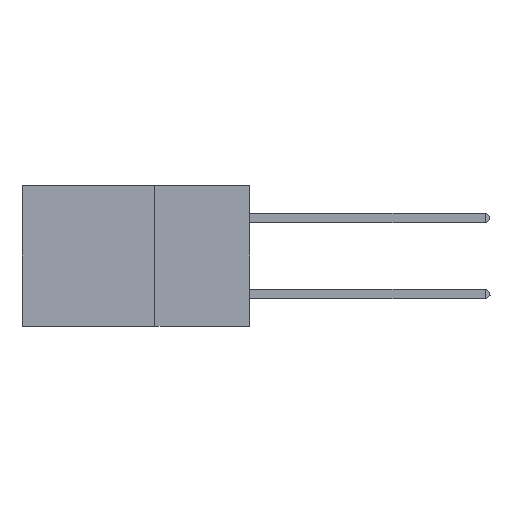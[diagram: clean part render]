
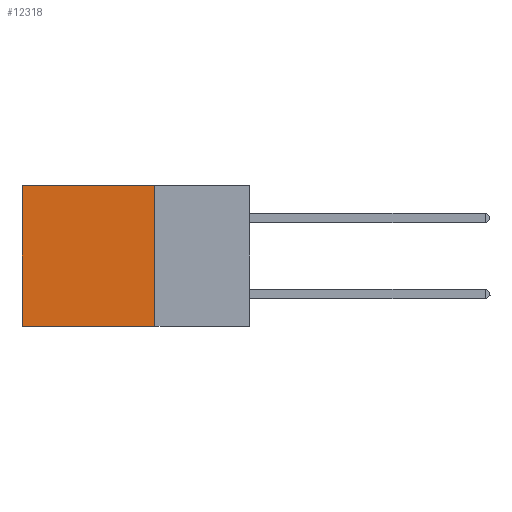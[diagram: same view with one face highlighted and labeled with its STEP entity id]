
A CAD part, left-side view. The second image highlights one B-rep face of the part: STEP entity #12318.
In plain terms, the highlighted planar face has unit normal (-1, 0, 0).
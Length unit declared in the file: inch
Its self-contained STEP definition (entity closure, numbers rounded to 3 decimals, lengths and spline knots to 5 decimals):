
#262 = CARTESIAN_POINT ( 'NONE',  ( 0.2875, 0.25, -0.37 ) ) ;
#1413 = CARTESIAN_POINT ( 'NONE',  ( 0.2875, 0.25, 0. ) ) ;
#1701 = DIRECTION ( 'NONE',  ( 1., 0., 0. ) ) ;
#1727 = VECTOR ( 'NONE', #26050, 39.37008 ) ;
#2191 = ORIENTED_EDGE ( 'NONE', *, *, #23558, .F. ) ;
#5407 = DIRECTION ( 'NONE',  ( 0., 1., 0. ) ) ;
#6178 = DIRECTION ( 'NONE',  ( 0., 1., 0. ) ) ;
#6446 = VECTOR ( 'NONE', #5407, 39.37008 ) ;
#7744 = FACE_OUTER_BOUND ( 'NONE', #20678, .T. ) ;
#8039 = DIRECTION ( 'NONE',  ( 0., 0., -1. ) ) ;
#8123 = VECTOR ( 'NONE', #6178, 39.37008 ) ;
#8472 = LINE ( 'NONE', #13001, #8123 ) ;
#8749 = EDGE_CURVE ( 'NONE', #18661, #9521, #18958, .T. ) ;
#9521 = VERTEX_POINT ( 'NONE', #22661 ) ;
#10892 = EDGE_CURVE ( 'NONE', #20650, #18661, #8472, .T. ) ;
#10921 = ORIENTED_EDGE ( 'NONE', *, *, #12912, .F. ) ;
#12318 = ADVANCED_FACE ( 'NONE', ( #7744 ), #20641, .F. ) ;
#12912 = EDGE_CURVE ( 'NONE', #20650, #13744, #21455, .T. ) ;
#13001 = CARTESIAN_POINT ( 'NONE',  ( 0.2875, 0.25, 0. ) ) ;
#13744 = VERTEX_POINT ( 'NONE', #262 ) ;
#14013 = CARTESIAN_POINT ( 'NONE',  ( 0.2875, 0.25, 0. ) ) ;
#14971 = DIRECTION ( 'NONE',  ( 0., 0., -1. ) ) ;
#15167 = CARTESIAN_POINT ( 'NONE',  ( 0.2875, 0.6, 0. ) ) ;
#15992 = CARTESIAN_POINT ( 'NONE',  ( 0.2875, 0.6, 0. ) ) ;
#16935 = ORIENTED_EDGE ( 'NONE', *, *, #8749, .T. ) ;
#18661 = VERTEX_POINT ( 'NONE', #15992 ) ;
#18842 = LINE ( 'NONE', #24756, #6446 ) ;
#18958 = LINE ( 'NONE', #15167, #19941 ) ;
#19941 = VECTOR ( 'NONE', #14971, 39.37008 ) ;
#20515 = AXIS2_PLACEMENT_3D ( 'NONE', #1413, #1701, #8039 ) ;
#20641 = PLANE ( 'NONE',  #20515 ) ;
#20650 = VERTEX_POINT ( 'NONE', #14013 ) ;
#20678 = EDGE_LOOP ( 'NONE', ( #16935, #2191, #10921, #22550 ) ) ;
#21455 = LINE ( 'NONE', #21772, #1727 ) ;
#21772 = CARTESIAN_POINT ( 'NONE',  ( 0.2875, 0.25, 0. ) ) ;
#22550 = ORIENTED_EDGE ( 'NONE', *, *, #10892, .T. ) ;
#22661 = CARTESIAN_POINT ( 'NONE',  ( 0.2875, 0.6, -0.37 ) ) ;
#23558 = EDGE_CURVE ( 'NONE', #13744, #9521, #18842, .T. ) ;
#24756 = CARTESIAN_POINT ( 'NONE',  ( 0.2875, 0.25, -0.37 ) ) ;
#26050 = DIRECTION ( 'NONE',  ( 0., 0., -1. ) ) ;
